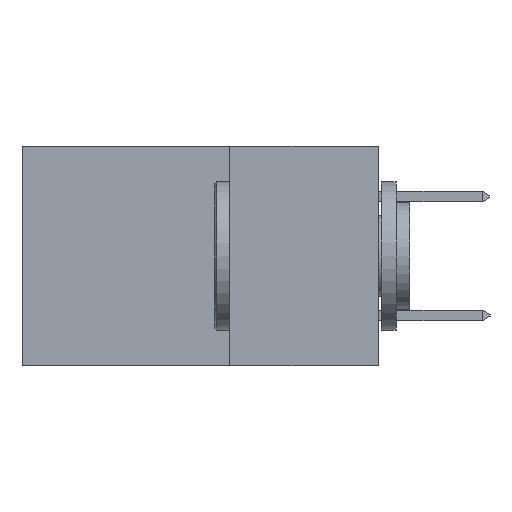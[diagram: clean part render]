
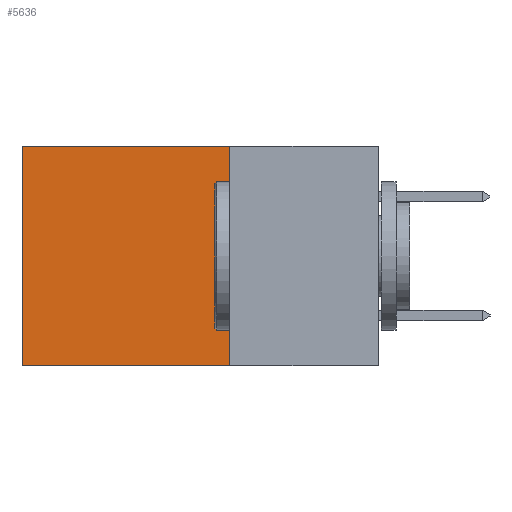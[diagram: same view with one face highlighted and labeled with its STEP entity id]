
A CAD part, left-side view. The second image highlights one B-rep face of the part: STEP entity #5636.
In plain terms, the highlighted planar face has unit normal (-1, 0, 0).
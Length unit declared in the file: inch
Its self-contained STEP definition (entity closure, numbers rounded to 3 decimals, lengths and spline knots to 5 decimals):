
#840 = LINE ( 'NONE', #6595, #8684 ) ;
#1350 = EDGE_LOOP ( 'NONE', ( #4195, #7597, #4617, #6842 ) ) ;
#1364 = VECTOR ( 'NONE', #5082, 39.37008 ) ;
#2494 = LINE ( 'NONE', #8472, #7820 ) ;
#2766 = VERTEX_POINT ( 'NONE', #7327 ) ;
#3066 = VERTEX_POINT ( 'NONE', #3570 ) ;
#3570 = CARTESIAN_POINT ( 'NONE',  ( 0.2615, 0.25, 0. ) ) ;
#3735 = VECTOR ( 'NONE', #6607, 39.37008 ) ;
#4135 = EDGE_CURVE ( 'NONE', #12179, #2766, #13370, .T. ) ;
#4195 = ORIENTED_EDGE ( 'NONE', *, *, #4135, .T. ) ;
#4617 = ORIENTED_EDGE ( 'NONE', *, *, #9281, .F. ) ;
#5082 = DIRECTION ( 'NONE',  ( 0., 0., -1. ) ) ;
#5282 = DIRECTION ( 'NONE',  ( 0., 1., 0. ) ) ;
#5302 = CARTESIAN_POINT ( 'NONE',  ( 0.2615, 0.25, -0.37 ) ) ;
#5636 = ADVANCED_FACE ( 'NONE', ( #6657 ), #8847, .F. ) ;
#6595 = CARTESIAN_POINT ( 'NONE',  ( 0.2615, 0.25, -0.37 ) ) ;
#6607 = DIRECTION ( 'NONE',  ( 0., 0., -1. ) ) ;
#6657 = FACE_OUTER_BOUND ( 'NONE', #1350, .T. ) ;
#6783 = CARTESIAN_POINT ( 'NONE',  ( 0.2615, 0.6, -0.37 ) ) ;
#6842 = ORIENTED_EDGE ( 'NONE', *, *, #10612, .T. ) ;
#7327 = CARTESIAN_POINT ( 'NONE',  ( 0.2615, 0.6, -0.37 ) ) ;
#7597 = ORIENTED_EDGE ( 'NONE', *, *, #9115, .F. ) ;
#7791 = AXIS2_PLACEMENT_3D ( 'NONE', #9109, #8820, #8808 ) ;
#7820 = VECTOR ( 'NONE', #5282, 39.37008 ) ;
#8472 = CARTESIAN_POINT ( 'NONE',  ( 0.2615, 0.25, 0. ) ) ;
#8684 = VECTOR ( 'NONE', #10664, 39.37008 ) ;
#8808 = DIRECTION ( 'NONE',  ( 0., 0., -1. ) ) ;
#8820 = DIRECTION ( 'NONE',  ( 1., 0., 0. ) ) ;
#8847 = PLANE ( 'NONE',  #7791 ) ;
#8871 = CARTESIAN_POINT ( 'NONE',  ( 0.2615, 0.6, 0. ) ) ;
#9109 = CARTESIAN_POINT ( 'NONE',  ( 0.2615, 0.25, -0.37 ) ) ;
#9115 = EDGE_CURVE ( 'NONE', #9446, #2766, #840, .T. ) ;
#9281 = EDGE_CURVE ( 'NONE', #3066, #9446, #9453, .T. ) ;
#9446 = VERTEX_POINT ( 'NONE', #5302 ) ;
#9453 = LINE ( 'NONE', #11288, #1364 ) ;
#10612 = EDGE_CURVE ( 'NONE', #3066, #12179, #2494, .T. ) ;
#10664 = DIRECTION ( 'NONE',  ( 0., 1., 0. ) ) ;
#11288 = CARTESIAN_POINT ( 'NONE',  ( 0.2615, 0.25, -0.37 ) ) ;
#12179 = VERTEX_POINT ( 'NONE', #8871 ) ;
#13370 = LINE ( 'NONE', #6783, #3735 ) ;
